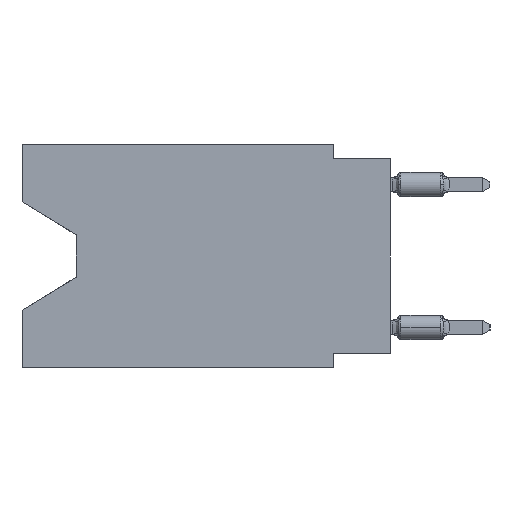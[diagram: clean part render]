
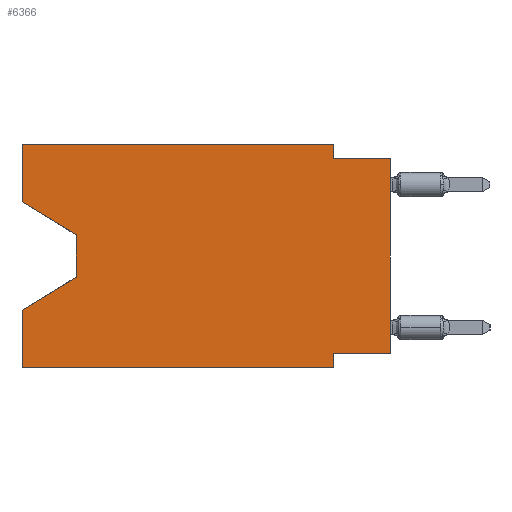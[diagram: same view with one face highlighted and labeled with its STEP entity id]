
A CAD part, left-side view. The second image highlights one B-rep face of the part: STEP entity #6366.
In plain terms, the highlighted planar face has unit normal (-1, 0, 0).
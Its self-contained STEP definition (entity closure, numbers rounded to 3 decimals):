
#336 = CARTESIAN_POINT ( 'NONE',  ( 0., 13.97, -4.013 ) ) ;
#442 = CARTESIAN_POINT ( 'NONE',  ( 0., 0., -9.271 ) ) ;
#556 = DIRECTION ( 'NONE',  ( 0., -1., 0. ) ) ;
#2310 = ORIENTED_EDGE ( 'NONE', *, *, #3535, .T. ) ;
#2397 = DIRECTION ( 'NONE',  ( 0., -1., 0. ) ) ;
#2670 = CARTESIAN_POINT ( 'NONE',  ( 0., 13.97, -5.893 ) ) ;
#2825 = LINE ( 'NONE', #16756, #39946 ) ;
#2960 = VERTEX_POINT ( 'NONE', #31416 ) ;
#3347 = LINE ( 'NONE', #34428, #32683 ) ;
#3535 = EDGE_CURVE ( 'NONE', #29681, #23067, #30968, .T. ) ;
#3768 = VECTOR ( 'NONE', #41391, 1000. ) ;
#3870 = LINE ( 'NONE', #442, #3768 ) ;
#3949 = DIRECTION ( 'NONE',  ( 0., 0., -1. ) ) ;
#4926 = ORIENTED_EDGE ( 'NONE', *, *, #8633, .F. ) ;
#5327 = VECTOR ( 'NONE', #16622, 1000. ) ;
#5407 = ORIENTED_EDGE ( 'NONE', *, *, #29142, .T. ) ;
#6086 = AXIS2_PLACEMENT_3D ( 'NONE', #31846, #11690, #3949 ) ;
#6366 = ADVANCED_FACE ( 'NONE', ( #8255 ), #14465, .F. ) ;
#7118 = CARTESIAN_POINT ( 'NONE',  ( 0., 0., -9.271 ) ) ;
#7225 = CARTESIAN_POINT ( 'NONE',  ( 0., 16.383, -7.36 ) ) ;
#7931 = ORIENTED_EDGE ( 'NONE', *, *, #41573, .T. ) ;
#8255 = FACE_OUTER_BOUND ( 'NONE', #10888, .T. ) ;
#8578 = VERTEX_POINT ( 'NONE', #26944 ) ;
#8633 = EDGE_CURVE ( 'NONE', #31591, #23067, #20085, .T. ) ;
#9139 = LINE ( 'NONE', #23090, #22336 ) ;
#9267 = LINE ( 'NONE', #41035, #41564 ) ;
#9823 = DIRECTION ( 'NONE',  ( 0., 0., -1. ) ) ;
#9990 = CARTESIAN_POINT ( 'NONE',  ( 0., 16.383, -2.546 ) ) ;
#10888 = EDGE_LOOP ( 'NONE', ( #5407, #18343, #2310, #4926, #16320, #17019, #37009, #7931, #44661, #44541, #38145, #34134 ) ) ;
#11064 = EDGE_CURVE ( 'NONE', #29998, #23493, #3870, .T. ) ;
#11150 = EDGE_CURVE ( 'NONE', #31591, #8578, #39411, .T. ) ;
#11690 = DIRECTION ( 'NONE',  ( 1., 0., 0. ) ) ;
#12667 = VERTEX_POINT ( 'NONE', #18103 ) ;
#13891 = VECTOR ( 'NONE', #14047, 1000. ) ;
#14047 = DIRECTION ( 'NONE',  ( 0., 0.855, -0.519 ) ) ;
#14465 = PLANE ( 'NONE',  #6086 ) ;
#14953 = EDGE_CURVE ( 'NONE', #27834, #29681, #20690, .T. ) ;
#16320 = ORIENTED_EDGE ( 'NONE', *, *, #11150, .T. ) ;
#16563 = DIRECTION ( 'NONE',  ( 0., 0., 1. ) ) ;
#16622 = DIRECTION ( 'NONE',  ( 0., 0., 1. ) ) ;
#16756 = CARTESIAN_POINT ( 'NONE',  ( 0., 2.54, -9.906 ) ) ;
#16819 = CARTESIAN_POINT ( 'NONE',  ( 0., 16.383, 0. ) ) ;
#17019 = ORIENTED_EDGE ( 'NONE', *, *, #43458, .F. ) ;
#18103 = CARTESIAN_POINT ( 'NONE',  ( 0., 0., -0.635 ) ) ;
#18343 = ORIENTED_EDGE ( 'NONE', *, *, #14953, .T. ) ;
#18978 = CARTESIAN_POINT ( 'NONE',  ( 0., 16.383, 0. ) ) ;
#19776 = VERTEX_POINT ( 'NONE', #36700 ) ;
#20085 = LINE ( 'NONE', #36778, #35290 ) ;
#20531 = VECTOR ( 'NONE', #556, 1000. ) ;
#20690 = LINE ( 'NONE', #336, #29589 ) ;
#20717 = EDGE_CURVE ( 'NONE', #24684, #23128, #36136, .T. ) ;
#21168 = EDGE_CURVE ( 'NONE', #19776, #12667, #43597, .T. ) ;
#22336 = VECTOR ( 'NONE', #23532, 1000. ) ;
#23067 = VERTEX_POINT ( 'NONE', #7225 ) ;
#23090 = CARTESIAN_POINT ( 'NONE',  ( 0., 16.383, -2.546 ) ) ;
#23128 = VERTEX_POINT ( 'NONE', #16819 ) ;
#23493 = VERTEX_POINT ( 'NONE', #44919 ) ;
#23532 = DIRECTION ( 'NONE',  ( 0., -0.855, -0.519 ) ) ;
#24684 = VERTEX_POINT ( 'NONE', #9990 ) ;
#26944 = CARTESIAN_POINT ( 'NONE',  ( 0., 2.54, -9.906 ) ) ;
#27834 = VERTEX_POINT ( 'NONE', #30769 ) ;
#28445 = CARTESIAN_POINT ( 'NONE',  ( 0., 16.383, -9.906 ) ) ;
#29142 = EDGE_CURVE ( 'NONE', #24684, #27834, #9139, .T. ) ;
#29589 = VECTOR ( 'NONE', #31207, 1000. ) ;
#29681 = VERTEX_POINT ( 'NONE', #2670 ) ;
#29998 = VERTEX_POINT ( 'NONE', #7118 ) ;
#30376 = DIRECTION ( 'NONE',  ( 0., 0., 1. ) ) ;
#30769 = CARTESIAN_POINT ( 'NONE',  ( 0., 13.97, -4.013 ) ) ;
#30968 = LINE ( 'NONE', #44493, #13891 ) ;
#31062 = VECTOR ( 'NONE', #9823, 1000. ) ;
#31082 = LINE ( 'NONE', #45041, #31062 ) ;
#31207 = DIRECTION ( 'NONE',  ( 0., 0., -1. ) ) ;
#31416 = CARTESIAN_POINT ( 'NONE',  ( 0., 2.54, 0. ) ) ;
#31591 = VERTEX_POINT ( 'NONE', #39379 ) ;
#31846 = CARTESIAN_POINT ( 'NONE',  ( 0., 16.383, 0. ) ) ;
#32370 = VECTOR ( 'NONE', #2397, 1000. ) ;
#32683 = VECTOR ( 'NONE', #38086, 1000. ) ;
#34134 = ORIENTED_EDGE ( 'NONE', *, *, #20717, .F. ) ;
#34428 = CARTESIAN_POINT ( 'NONE',  ( 0., 16.383, 0. ) ) ;
#35290 = VECTOR ( 'NONE', #30376, 1000. ) ;
#36136 = LINE ( 'NONE', #18978, #5327 ) ;
#36700 = CARTESIAN_POINT ( 'NONE',  ( 0., 2.54, -0.635 ) ) ;
#36778 = CARTESIAN_POINT ( 'NONE',  ( 0., 16.383, 0. ) ) ;
#36948 = CARTESIAN_POINT ( 'NONE',  ( 0., 0., -0.635 ) ) ;
#37009 = ORIENTED_EDGE ( 'NONE', *, *, #11064, .F. ) ;
#38086 = DIRECTION ( 'NONE',  ( 0., -1., 0. ) ) ;
#38145 = ORIENTED_EDGE ( 'NONE', *, *, #44612, .F. ) ;
#39379 = CARTESIAN_POINT ( 'NONE',  ( 0., 16.383, -9.906 ) ) ;
#39411 = LINE ( 'NONE', #28445, #20531 ) ;
#39946 = VECTOR ( 'NONE', #42153, 1000. ) ;
#41035 = CARTESIAN_POINT ( 'NONE',  ( 0., 0., 0. ) ) ;
#41391 = DIRECTION ( 'NONE',  ( 0., 1., 0. ) ) ;
#41564 = VECTOR ( 'NONE', #16563, 1000. ) ;
#41573 = EDGE_CURVE ( 'NONE', #29998, #12667, #9267, .T. ) ;
#42055 = EDGE_CURVE ( 'NONE', #2960, #19776, #31082, .T. ) ;
#42153 = DIRECTION ( 'NONE',  ( 0., 0., -1. ) ) ;
#43458 = EDGE_CURVE ( 'NONE', #23493, #8578, #2825, .T. ) ;
#43597 = LINE ( 'NONE', #36948, #32370 ) ;
#44493 = CARTESIAN_POINT ( 'NONE',  ( 0., 13.97, -5.893 ) ) ;
#44541 = ORIENTED_EDGE ( 'NONE', *, *, #42055, .F. ) ;
#44612 = EDGE_CURVE ( 'NONE', #23128, #2960, #3347, .T. ) ;
#44661 = ORIENTED_EDGE ( 'NONE', *, *, #21168, .F. ) ;
#44919 = CARTESIAN_POINT ( 'NONE',  ( 0., 2.54, -9.271 ) ) ;
#45041 = CARTESIAN_POINT ( 'NONE',  ( 0., 2.54, 0. ) ) ;
